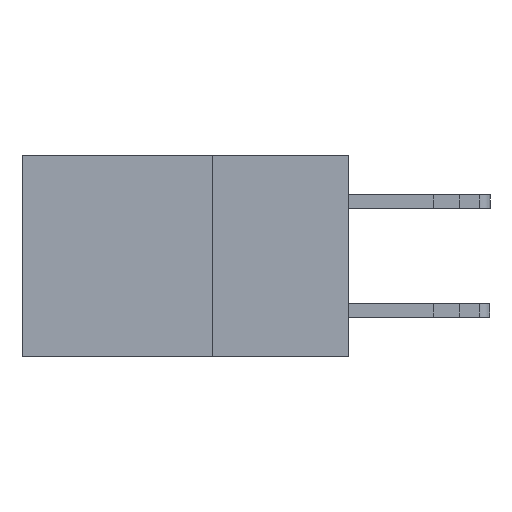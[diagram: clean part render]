
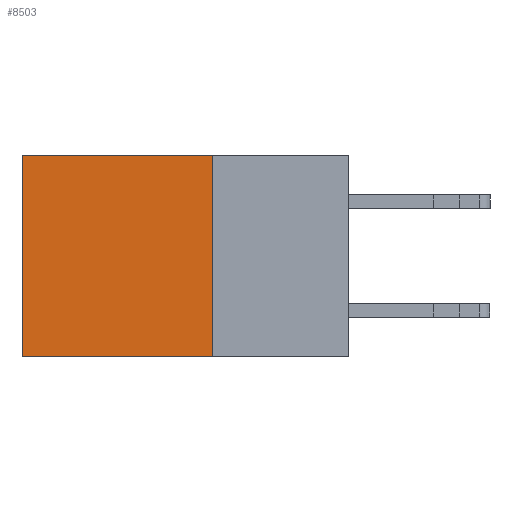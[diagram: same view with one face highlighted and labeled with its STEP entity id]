
A CAD part, left-side view. The second image highlights one B-rep face of the part: STEP entity #8503.
In plain terms, the highlighted planar face has unit normal (-1, 0, 0).
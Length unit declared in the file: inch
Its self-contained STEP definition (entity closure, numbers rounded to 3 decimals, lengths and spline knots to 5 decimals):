
#12 = EDGE_CURVE ( 'NONE', #9804, #956, #7281, .T. ) ;
#526 = CARTESIAN_POINT ( 'NONE',  ( 0.298, 0.25, 0. ) ) ;
#528 = VECTOR ( 'NONE', #4254, 39.37008 ) ;
#768 = LINE ( 'NONE', #2638, #8441 ) ;
#956 = VERTEX_POINT ( 'NONE', #2058 ) ;
#1319 = VECTOR ( 'NONE', #8079, 39.37008 ) ;
#1364 = DIRECTION ( 'NONE',  ( 0., 0., -1. ) ) ;
#2058 = CARTESIAN_POINT ( 'NONE',  ( 0.298, 0.6, 0. ) ) ;
#2638 = CARTESIAN_POINT ( 'NONE',  ( 0.298, 0.25, -0.37 ) ) ;
#3654 = CARTESIAN_POINT ( 'NONE',  ( 0.298, 0.6, -0.37 ) ) ;
#3699 = DIRECTION ( 'NONE',  ( 0., 1., 0. ) ) ;
#4012 = EDGE_CURVE ( 'NONE', #9804, #5965, #9451, .T. ) ;
#4254 = DIRECTION ( 'NONE',  ( 0., 0., -1. ) ) ;
#4622 = ORIENTED_EDGE ( 'NONE', *, *, #8693, .T. ) ;
#4873 = ORIENTED_EDGE ( 'NONE', *, *, #12, .T. ) ;
#5147 = CARTESIAN_POINT ( 'NONE',  ( 0.298, 0.25, 0. ) ) ;
#5350 = EDGE_LOOP ( 'NONE', ( #4622, #6537, #11635, #4873 ) ) ;
#5367 = CARTESIAN_POINT ( 'NONE',  ( 0.298, 0.6, 0. ) ) ;
#5512 = DIRECTION ( 'NONE',  ( 0., 1., 0. ) ) ;
#5965 = VERTEX_POINT ( 'NONE', #6333 ) ;
#6005 = CARTESIAN_POINT ( 'NONE',  ( 0.298, 0.25, 0. ) ) ;
#6111 = EDGE_CURVE ( 'NONE', #5965, #7572, #768, .T. ) ;
#6333 = CARTESIAN_POINT ( 'NONE',  ( 0.298, 0.25, -0.37 ) ) ;
#6361 = AXIS2_PLACEMENT_3D ( 'NONE', #6005, #6919, #1364 ) ;
#6537 = ORIENTED_EDGE ( 'NONE', *, *, #6111, .F. ) ;
#6919 = DIRECTION ( 'NONE',  ( 1., 0., 0. ) ) ;
#7281 = LINE ( 'NONE', #526, #9647 ) ;
#7572 = VERTEX_POINT ( 'NONE', #3654 ) ;
#7936 = FACE_OUTER_BOUND ( 'NONE', #5350, .T. ) ;
#8020 = CARTESIAN_POINT ( 'NONE',  ( 0.298, 0.25, 0. ) ) ;
#8079 = DIRECTION ( 'NONE',  ( 0., 0., -1. ) ) ;
#8441 = VECTOR ( 'NONE', #3699, 39.37008 ) ;
#8503 = ADVANCED_FACE ( 'NONE', ( #7936 ), #11328, .F. ) ;
#8693 = EDGE_CURVE ( 'NONE', #956, #7572, #10719, .T. ) ;
#9451 = LINE ( 'NONE', #8020, #528 ) ;
#9647 = VECTOR ( 'NONE', #5512, 39.37008 ) ;
#9804 = VERTEX_POINT ( 'NONE', #5147 ) ;
#10719 = LINE ( 'NONE', #5367, #1319 ) ;
#11328 = PLANE ( 'NONE',  #6361 ) ;
#11635 = ORIENTED_EDGE ( 'NONE', *, *, #4012, .F. ) ;
